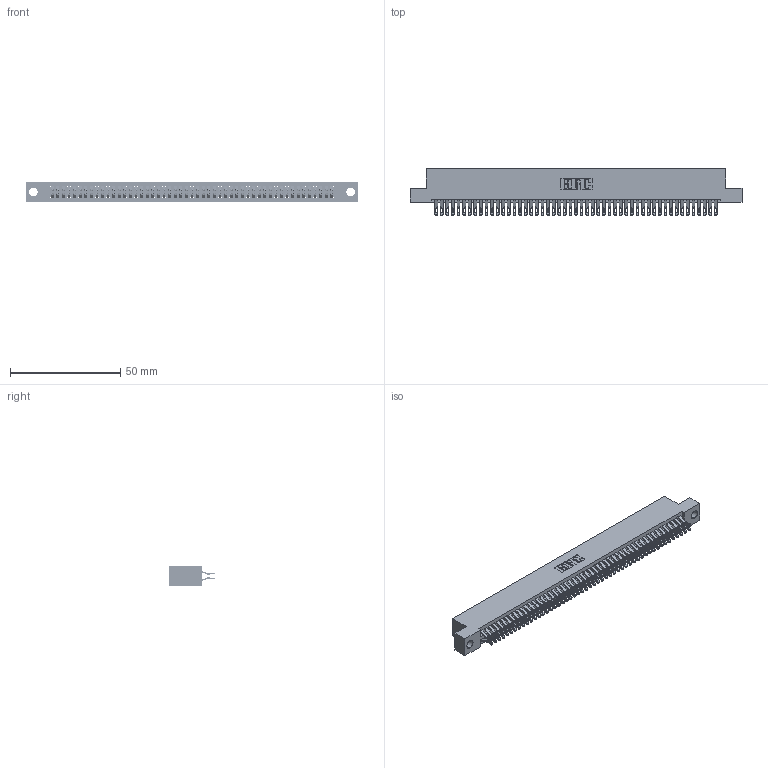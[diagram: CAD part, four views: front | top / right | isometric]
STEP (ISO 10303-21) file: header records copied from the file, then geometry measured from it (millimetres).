
FILE_DESCRIPTION (( 'STEP AP203' ), '1' );
FILE_NAME ('395-102-555-204.STEP', '2021-06-17T15:40:53', ( '' ), ( '' ), 'SwSTEP 2.0', 'SolidWorks 2020', '' );
FILE_SCHEMA (( 'CONFIG_CONTROL_DESIGN' ));
Length unit declared in the file: inch
Products named in the file (3): 345 Part_Flush Mounting Lugs - 0.156 Dia-TI; 345-292-001_555 Tail; 395-102-555-204
Assembly tree (103 placements, depth 2):
  395-102-555-204
    345 Part_Flush Mounting Lugs - 0.156 Dia-TI
    345-292-001_555 Tail  x102
Bounding box: 150.75 x 21.13 x 9.4 mm (x, y, z)
Volume: 14917.4 mm3; surface area: 23105.3 mm2
Topology: 103 solids, 103 shells, 5852 faces, 18431 edges, 12286 vertices
Faces by surface type: plane 3256, cylinder 2596
Entity records: 39549 total; most frequent: CARTESIAN_POINT 6660, ORIENTED_EDGE 6562, DIRECTION 5829, EDGE_CURVE 3281, VECTOR 2925, LINE 2925, VERTEX_POINT 2186, AXIS2_PLACEMENT_3D 1452
